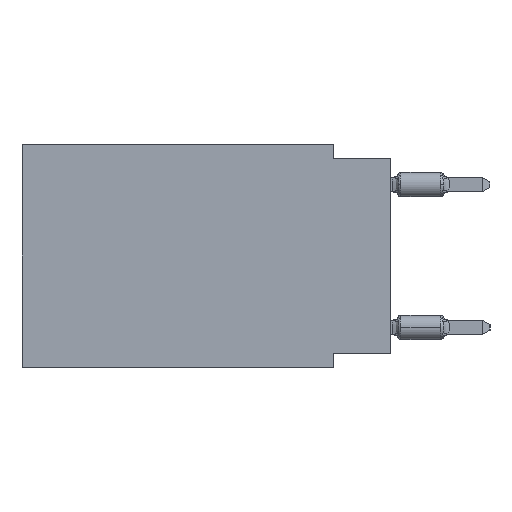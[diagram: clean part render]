
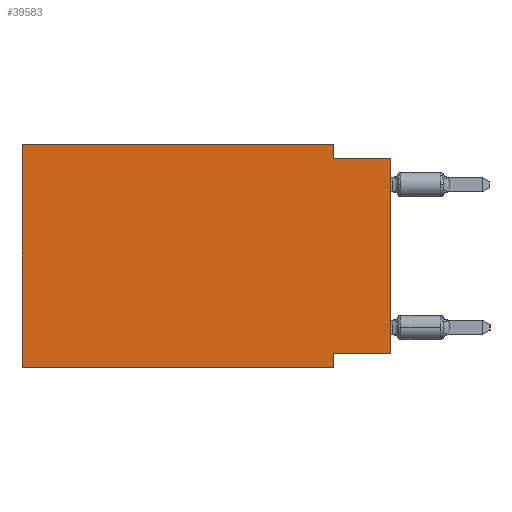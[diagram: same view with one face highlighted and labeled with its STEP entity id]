
A CAD part, left-side view. The second image highlights one B-rep face of the part: STEP entity #39583.
In plain terms, the highlighted planar face has unit normal (-1, 0, 0).
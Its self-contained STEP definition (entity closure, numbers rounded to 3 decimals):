
#317 = VERTEX_POINT ( 'NONE', #6926 ) ;
#564 = LINE ( 'NONE', #27464, #27177 ) ;
#816 = CARTESIAN_POINT ( 'NONE',  ( 0., 16.383, 0. ) ) ;
#2660 = VERTEX_POINT ( 'NONE', #54392 ) ;
#2733 = LINE ( 'NONE', #15876, #36738 ) ;
#3401 = ORIENTED_EDGE ( 'NONE', *, *, #40626, .F. ) ;
#4653 = DIRECTION ( 'NONE',  ( 0., 0., 1. ) ) ;
#4874 = VECTOR ( 'NONE', #30555, 1000. ) ;
#5034 = LINE ( 'NONE', #23744, #23064 ) ;
#5421 = CARTESIAN_POINT ( 'NONE',  ( 0., 0., -0.635 ) ) ;
#5512 = EDGE_CURVE ( 'NONE', #2660, #6967, #5034, .T. ) ;
#6432 = DIRECTION ( 'NONE',  ( 0., 0., -1. ) ) ;
#6926 = CARTESIAN_POINT ( 'NONE',  ( 0., 2.54, -9.271 ) ) ;
#6967 = VERTEX_POINT ( 'NONE', #52978 ) ;
#7249 = ORIENTED_EDGE ( 'NONE', *, *, #37005, .F. ) ;
#7734 = VECTOR ( 'NONE', #8835, 1000. ) ;
#8766 = ORIENTED_EDGE ( 'NONE', *, *, #5512, .T. ) ;
#8835 = DIRECTION ( 'NONE',  ( 0., 1., 0. ) ) ;
#9113 = CARTESIAN_POINT ( 'NONE',  ( 0., 0., -9.271 ) ) ;
#14592 = EDGE_LOOP ( 'NONE', ( #8766, #54980, #7249, #3401, #34141, #25207, #50091, #44947 ) ) ;
#14635 = CARTESIAN_POINT ( 'NONE',  ( 0., 2.54, -9.906 ) ) ;
#15876 = CARTESIAN_POINT ( 'NONE',  ( 0., 16.383, -9.906 ) ) ;
#16667 = VERTEX_POINT ( 'NONE', #37597 ) ;
#18278 = VECTOR ( 'NONE', #50187, 1000. ) ;
#20987 = CARTESIAN_POINT ( 'NONE',  ( 0., 16.383, 0. ) ) ;
#22405 = LINE ( 'NONE', #5421, #18278 ) ;
#22686 = CARTESIAN_POINT ( 'NONE',  ( 0., 16.383, 0. ) ) ;
#23064 = VECTOR ( 'NONE', #23164, 1000. ) ;
#23164 = DIRECTION ( 'NONE',  ( 0., 0., 1. ) ) ;
#23744 = CARTESIAN_POINT ( 'NONE',  ( 0., 0., 0. ) ) ;
#24861 = LINE ( 'NONE', #14635, #33353 ) ;
#25207 = ORIENTED_EDGE ( 'NONE', *, *, #26330, .T. ) ;
#25213 = EDGE_CURVE ( 'NONE', #2660, #317, #26693, .T. ) ;
#25673 = DIRECTION ( 'NONE',  ( 1., 0., 0. ) ) ;
#25965 = DIRECTION ( 'NONE',  ( 0., 0., -1. ) ) ;
#26164 = CARTESIAN_POINT ( 'NONE',  ( 0., 2.54, 0. ) ) ;
#26330 = EDGE_CURVE ( 'NONE', #28892, #16667, #2733, .T. ) ;
#26693 = LINE ( 'NONE', #9113, #7734 ) ;
#27177 = VECTOR ( 'NONE', #4653, 1000. ) ;
#27464 = CARTESIAN_POINT ( 'NONE',  ( 0., 16.383, 0. ) ) ;
#28888 = EDGE_CURVE ( 'NONE', #46450, #6967, #22405, .T. ) ;
#28892 = VERTEX_POINT ( 'NONE', #44930 ) ;
#29643 = DIRECTION ( 'NONE',  ( 0., -1., 0. ) ) ;
#30555 = DIRECTION ( 'NONE',  ( 0., 0., -1. ) ) ;
#30611 = LINE ( 'NONE', #22686, #48022 ) ;
#33353 = VECTOR ( 'NONE', #6432, 1000. ) ;
#33808 = EDGE_CURVE ( 'NONE', #28892, #36701, #564, .T. ) ;
#34141 = ORIENTED_EDGE ( 'NONE', *, *, #33808, .F. ) ;
#34453 = VERTEX_POINT ( 'NONE', #55738 ) ;
#36701 = VERTEX_POINT ( 'NONE', #816 ) ;
#36738 = VECTOR ( 'NONE', #29643, 1000. ) ;
#37005 = EDGE_CURVE ( 'NONE', #34453, #46450, #53066, .T. ) ;
#37597 = CARTESIAN_POINT ( 'NONE',  ( 0., 2.54, -9.906 ) ) ;
#39108 = FACE_OUTER_BOUND ( 'NONE', #14592, .T. ) ;
#39583 = ADVANCED_FACE ( 'NONE', ( #39108 ), #39700, .F. ) ;
#39700 = PLANE ( 'NONE',  #52753 ) ;
#40626 = EDGE_CURVE ( 'NONE', #36701, #34453, #30611, .T. ) ;
#44930 = CARTESIAN_POINT ( 'NONE',  ( 0., 16.383, -9.906 ) ) ;
#44947 = ORIENTED_EDGE ( 'NONE', *, *, #25213, .F. ) ;
#46299 = EDGE_CURVE ( 'NONE', #317, #16667, #24861, .T. ) ;
#46450 = VERTEX_POINT ( 'NONE', #57018 ) ;
#48022 = VECTOR ( 'NONE', #49885, 1000. ) ;
#49885 = DIRECTION ( 'NONE',  ( 0., -1., 0. ) ) ;
#50091 = ORIENTED_EDGE ( 'NONE', *, *, #46299, .F. ) ;
#50187 = DIRECTION ( 'NONE',  ( 0., -1., 0. ) ) ;
#52753 = AXIS2_PLACEMENT_3D ( 'NONE', #20987, #25673, #25965 ) ;
#52978 = CARTESIAN_POINT ( 'NONE',  ( 0., 0., -0.635 ) ) ;
#53066 = LINE ( 'NONE', #26164, #4874 ) ;
#54392 = CARTESIAN_POINT ( 'NONE',  ( 0., 0., -9.271 ) ) ;
#54980 = ORIENTED_EDGE ( 'NONE', *, *, #28888, .F. ) ;
#55738 = CARTESIAN_POINT ( 'NONE',  ( 0., 2.54, 0. ) ) ;
#57018 = CARTESIAN_POINT ( 'NONE',  ( 0., 2.54, -0.635 ) ) ;
